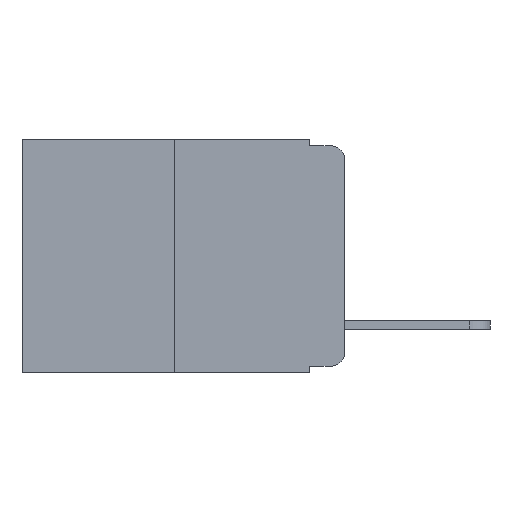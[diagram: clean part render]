
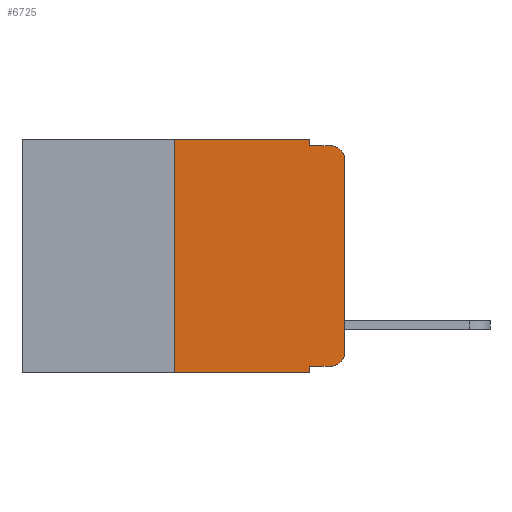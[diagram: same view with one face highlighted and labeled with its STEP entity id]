
A CAD part, left-side view. The second image highlights one B-rep face of the part: STEP entity #6725.
In plain terms, the highlighted planar face has unit normal (-1, 0, 0).
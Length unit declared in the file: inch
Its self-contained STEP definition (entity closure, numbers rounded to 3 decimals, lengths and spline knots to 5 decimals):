
#14 = DIRECTION ( 'NONE',  ( 1., 0., 0. ) ) ;
#267 = VECTOR ( 'NONE', #5405, 39.37008 ) ;
#582 = CARTESIAN_POINT ( 'NONE',  ( 0., 0.25, 0. ) ) ;
#653 = VECTOR ( 'NONE', #4574, 39.37008 ) ;
#719 = ORIENTED_EDGE ( 'NONE', *, *, #5200, .T. ) ;
#833 = PLANE ( 'NONE',  #16081 ) ;
#1043 = ORIENTED_EDGE ( 'NONE', *, *, #16235, .T. ) ;
#1475 = LINE ( 'NONE', #12478, #1971 ) ;
#1971 = VECTOR ( 'NONE', #6148, 39.37008 ) ;
#2722 = DIRECTION ( 'NONE',  ( 0., 0., 1. ) ) ;
#3045 = CARTESIAN_POINT ( 'NONE',  ( 0., 0.02, -0.333 ) ) ;
#3176 = FACE_OUTER_BOUND ( 'NONE', #16639, .T. ) ;
#3549 = CARTESIAN_POINT ( 'NONE',  ( 0., 0.473, -0.343 ) ) ;
#3968 = ORIENTED_EDGE ( 'NONE', *, *, #14966, .F. ) ;
#3973 = CARTESIAN_POINT ( 'NONE',  ( 0., 0.051, -0.333 ) ) ;
#4141 = VECTOR ( 'NONE', #2722, 39.37008 ) ;
#4331 = EDGE_CURVE ( 'NONE', #16071, #19641, #1475, .T. ) ;
#4574 = DIRECTION ( 'NONE',  ( 0., -1., 0. ) ) ;
#4644 = LINE ( 'NONE', #7230, #4141 ) ;
#4789 = EDGE_CURVE ( 'NONE', #16045, #16071, #4644, .T. ) ;
#5086 = DIRECTION ( 'NONE',  ( 0., 0., -1. ) ) ;
#5200 = EDGE_CURVE ( 'NONE', #18965, #8997, #7872, .T. ) ;
#5226 = VERTEX_POINT ( 'NONE', #17256 ) ;
#5405 = DIRECTION ( 'NONE',  ( 0., -1., 0. ) ) ;
#6148 = DIRECTION ( 'NONE',  ( 0., -1., 0. ) ) ;
#6217 = DIRECTION ( 'NONE',  ( 0., 0., -1. ) ) ;
#6264 = LINE ( 'NONE', #15853, #8967 ) ;
#6725 = ADVANCED_FACE ( 'NONE', ( #3176 ), #833, .F. ) ;
#7230 = CARTESIAN_POINT ( 'NONE',  ( 0., 0.25, 0. ) ) ;
#7268 = CARTESIAN_POINT ( 'NONE',  ( 0., 0.473, 0. ) ) ;
#7434 = VECTOR ( 'NONE', #15479, 39.37008 ) ;
#7763 = EDGE_CURVE ( 'NONE', #9447, #18965, #12006, .T. ) ;
#7872 = CIRCLE ( 'NONE', #9660, 0.02 ) ;
#8878 = ORIENTED_EDGE ( 'NONE', *, *, #15117, .F. ) ;
#8967 = VECTOR ( 'NONE', #5086, 39.37008 ) ;
#8997 = VERTEX_POINT ( 'NONE', #9220 ) ;
#9220 = CARTESIAN_POINT ( 'NONE',  ( 0., 0., -0.313 ) ) ;
#9364 = CARTESIAN_POINT ( 'NONE',  ( 0., 0.051, 0. ) ) ;
#9447 = VERTEX_POINT ( 'NONE', #3973 ) ;
#9660 = AXIS2_PLACEMENT_3D ( 'NONE', #15338, #10697, #6217 ) ;
#9806 = CARTESIAN_POINT ( 'NONE',  ( 0., 0.051, -0.01 ) ) ;
#9910 = DIRECTION ( 'NONE',  ( 0., 0., -1. ) ) ;
#10156 = LINE ( 'NONE', #3549, #267 ) ;
#10236 = EDGE_CURVE ( 'NONE', #19641, #16772, #6264, .T. ) ;
#10412 = EDGE_CURVE ( 'NONE', #11374, #11680, #10918, .T. ) ;
#10624 = CARTESIAN_POINT ( 'NONE',  ( 0., 0.051, -0.333 ) ) ;
#10694 = ORIENTED_EDGE ( 'NONE', *, *, #4331, .F. ) ;
#10697 = DIRECTION ( 'NONE',  ( -1., 0., 0. ) ) ;
#10918 = CIRCLE ( 'NONE', #18064, 0.02 ) ;
#11374 = VERTEX_POINT ( 'NONE', #15743 ) ;
#11680 = VERTEX_POINT ( 'NONE', #15175 ) ;
#11944 = CARTESIAN_POINT ( 'NONE',  ( 0., 0.02, -0.03 ) ) ;
#12006 = LINE ( 'NONE', #10624, #653 ) ;
#12282 = CARTESIAN_POINT ( 'NONE',  ( 0., 0.051, 0. ) ) ;
#12478 = CARTESIAN_POINT ( 'NONE',  ( 0., 0.473, 0. ) ) ;
#12801 = ORIENTED_EDGE ( 'NONE', *, *, #14664, .T. ) ;
#12964 = DIRECTION ( 'NONE',  ( 0., -1., 0. ) ) ;
#13078 = LINE ( 'NONE', #9806, #18679 ) ;
#13632 = CARTESIAN_POINT ( 'NONE',  ( 0., 0.051, -0.01 ) ) ;
#13792 = CARTESIAN_POINT ( 'NONE',  ( 0., 0., 0. ) ) ;
#13993 = DIRECTION ( 'NONE',  ( 0., 0., 1. ) ) ;
#14373 = ORIENTED_EDGE ( 'NONE', *, *, #10412, .T. ) ;
#14664 = EDGE_CURVE ( 'NONE', #16045, #5226, #10156, .T. ) ;
#14966 = EDGE_CURVE ( 'NONE', #9447, #5226, #16232, .T. ) ;
#15117 = EDGE_CURVE ( 'NONE', #16772, #11680, #13078, .T. ) ;
#15175 = CARTESIAN_POINT ( 'NONE',  ( 0., 0.02, -0.01 ) ) ;
#15338 = CARTESIAN_POINT ( 'NONE',  ( 0., 0.02, -0.313 ) ) ;
#15438 = VECTOR ( 'NONE', #13993, 39.37008 ) ;
#15479 = DIRECTION ( 'NONE',  ( 0., 0., -1. ) ) ;
#15549 = ORIENTED_EDGE ( 'NONE', *, *, #4789, .F. ) ;
#15743 = CARTESIAN_POINT ( 'NONE',  ( 0., 0., -0.03 ) ) ;
#15853 = CARTESIAN_POINT ( 'NONE',  ( 0., 0.051, 0. ) ) ;
#16045 = VERTEX_POINT ( 'NONE', #19477 ) ;
#16071 = VERTEX_POINT ( 'NONE', #582 ) ;
#16081 = AXIS2_PLACEMENT_3D ( 'NONE', #7268, #14, #20270 ) ;
#16232 = LINE ( 'NONE', #12282, #7434 ) ;
#16235 = EDGE_CURVE ( 'NONE', #8997, #11374, #20098, .T. ) ;
#16639 = EDGE_LOOP ( 'NONE', ( #1043, #14373, #8878, #19247, #10694, #15549, #12801, #3968, #17704, #719 ) ) ;
#16772 = VERTEX_POINT ( 'NONE', #13632 ) ;
#17256 = CARTESIAN_POINT ( 'NONE',  ( 0., 0.051, -0.343 ) ) ;
#17704 = ORIENTED_EDGE ( 'NONE', *, *, #7763, .T. ) ;
#18064 = AXIS2_PLACEMENT_3D ( 'NONE', #11944, #19265, #9910 ) ;
#18679 = VECTOR ( 'NONE', #12964, 39.37008 ) ;
#18965 = VERTEX_POINT ( 'NONE', #3045 ) ;
#19247 = ORIENTED_EDGE ( 'NONE', *, *, #10236, .F. ) ;
#19265 = DIRECTION ( 'NONE',  ( -1., 0., 0. ) ) ;
#19477 = CARTESIAN_POINT ( 'NONE',  ( 0., 0.25, -0.343 ) ) ;
#19641 = VERTEX_POINT ( 'NONE', #9364 ) ;
#20098 = LINE ( 'NONE', #13792, #15438 ) ;
#20270 = DIRECTION ( 'NONE',  ( 0., 0., -1. ) ) ;
